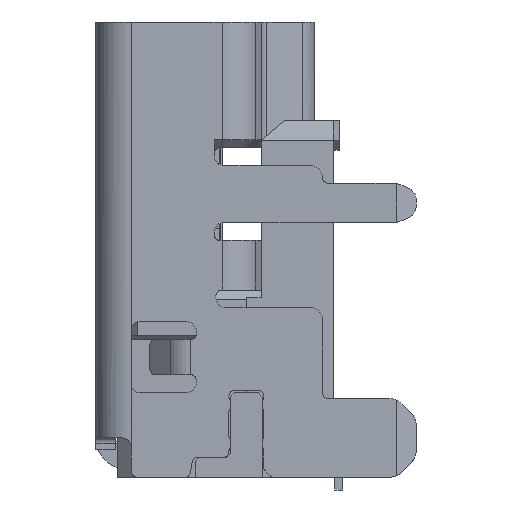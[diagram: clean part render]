
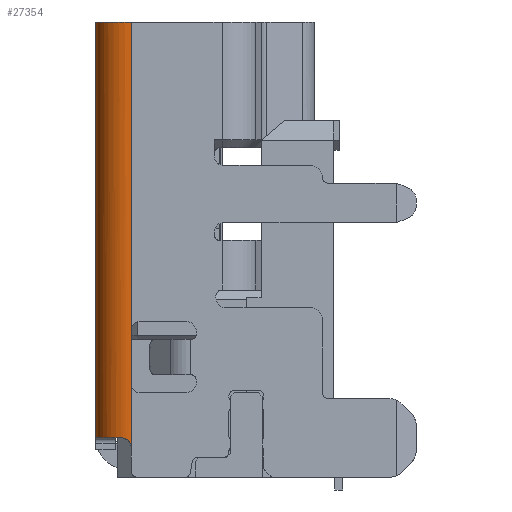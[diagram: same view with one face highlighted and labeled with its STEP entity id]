
A CAD part, left-side view. The second image highlights one B-rep face of the part: STEP entity #27354.
In plain terms, the highlighted cylindrical face has radius 0.9 mm (diameter 1.8 mm), a partial arc.
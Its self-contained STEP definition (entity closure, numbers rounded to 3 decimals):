
#1960 = DIRECTION ( 'NONE',  ( 0., 0., 1. ) ) ;
#2924 = VERTEX_POINT ( 'NONE', #66297 ) ;
#3146 = DIRECTION ( 'NONE',  ( 0., 0., -1. ) ) ;
#3292 = DIRECTION ( 'NONE',  ( 0., 0., -1. ) ) ;
#3440 = CARTESIAN_POINT ( 'NONE',  ( -7.5, -1.875, 2.42 ) ) ;
#4005 = AXIS2_PLACEMENT_3D ( 'NONE', #53851, #48777, #43670 ) ;
#4174 = CIRCLE ( 'NONE', #64042, 0.9 ) ;
#5714 = EDGE_CURVE ( 'NONE', #2924, #71550, #4174, .T. ) ;
#6759 = ORIENTED_EDGE ( 'NONE', *, *, #42271, .T. ) ;
#8764 = CARTESIAN_POINT ( 'NONE',  ( -7.5, -1.875, -1.005 ) ) ;
#10180 = EDGE_CURVE ( 'NONE', #45390, #64215, #56453, .T. ) ;
#12087 = CARTESIAN_POINT ( 'NONE',  ( -7.5, -1.875, 3.953 ) ) ;
#14672 = VECTOR ( 'NONE', #3146, 1000. ) ;
#15556 = VECTOR ( 'NONE', #62275, 1000. ) ;
#15806 = LINE ( 'NONE', #8764, #19588 ) ;
#19575 = CARTESIAN_POINT ( 'NONE',  ( -7.465, -2.125, 3.77 ) ) ;
#19588 = VECTOR ( 'NONE', #3292, 1000. ) ;
#20979 = DIRECTION ( 'NONE',  ( 0., 0., 1. ) ) ;
#22442 = CARTESIAN_POINT ( 'NONE',  ( -7.5, -1.875, 4.02 ) ) ;
#24005 = CIRCLE ( 'NONE', #4005, 0.9 ) ;
#25497 = CARTESIAN_POINT ( 'NONE',  ( -7.5, -1.875, -6.996 ) ) ;
#26940 = EDGE_CURVE ( 'NONE', #62517, #68354, #32882, .T. ) ;
#27354 = ADVANCED_FACE ( 'NONE', ( #62005 ), #57639, .T. ) ;
#28954 = CARTESIAN_POINT ( 'NONE',  ( -7.465, -2.125, 3.77 ) ) ;
#29230 = CARTESIAN_POINT ( 'NONE',  ( -6.6, -2.775, -6.78 ) ) ;
#29969 = ORIENTED_EDGE ( 'NONE', *, *, #5714, .T. ) ;
#30055 = DIRECTION ( 'NONE',  ( 0., 0., -1. ) ) ;
#31316 = ORIENTED_EDGE ( 'NONE', *, *, #49543, .T. ) ;
#32688 = CARTESIAN_POINT ( 'NONE',  ( -6.6, -1.875, -6.996 ) ) ;
#32882 = LINE ( 'NONE', #25497, #14672 ) ;
#33837 = DIRECTION ( 'NONE',  ( 1., 0., 0. ) ) ;
#35543 = CARTESIAN_POINT ( 'NONE',  ( -7.501, -1.903, 3.888 ) ) ;
#38303 = CARTESIAN_POINT ( 'NONE',  ( -6.6, -1.875, -6.78 ) ) ;
#39000 = EDGE_LOOP ( 'NONE', ( #59599, #59923, #70439, #31316, #29969, #6759, #40076 ) ) ;
#40076 = ORIENTED_EDGE ( 'NONE', *, *, #71233, .F. ) ;
#41010 = CARTESIAN_POINT ( 'NONE',  ( -7.483, -2.061, 3.77 ) ) ;
#42271 = EDGE_CURVE ( 'NONE', #71550, #43521, #44668, .T. ) ;
#43521 = VERTEX_POINT ( 'NONE', #47850 ) ;
#43670 = DIRECTION ( 'NONE',  ( 1., 0., 0. ) ) ;
#44668 = LINE ( 'NONE', #67747, #15556 ) ;
#45390 = VERTEX_POINT ( 'NONE', #19575 ) ;
#46478 = CARTESIAN_POINT ( 'NONE',  ( -7.5, -1.875, 4.02 ) ) ;
#47850 = CARTESIAN_POINT ( 'NONE',  ( -6.6, -2.775, 3.77 ) ) ;
#48777 = DIRECTION ( 'NONE',  ( 0., 0., 1. ) ) ;
#49543 = EDGE_CURVE ( 'NONE', #68354, #2924, #59683, .T. ) ;
#52723 = CARTESIAN_POINT ( 'NONE',  ( -7.493, -1.996, 3.796 ) ) ;
#53189 = AXIS2_PLACEMENT_3D ( 'NONE', #32688, #20979, #33837 ) ;
#53235 = VECTOR ( 'NONE', #30055, 1000. ) ;
#53851 = CARTESIAN_POINT ( 'NONE',  ( -6.6, -1.875, 3.77 ) ) ;
#56453 = B_SPLINE_CURVE_WITH_KNOTS ( 'NONE', 3,
 ( #28954, #41010, #52723, #35543, #12087, #46478 ),
 .UNSPECIFIED., .F., .F.,
 ( 4, 2, 4 ),
 ( 0., 0., 0. ),
 .UNSPECIFIED. ) ;
#57639 = CYLINDRICAL_SURFACE ( 'NONE', #53189, 0.9 ) ;
#58355 = CARTESIAN_POINT ( 'NONE',  ( -7.5, -1.875, 1.02 ) ) ;
#59599 = ORIENTED_EDGE ( 'NONE', *, *, #10180, .T. ) ;
#59683 = LINE ( 'NONE', #66338, #53235 ) ;
#59923 = ORIENTED_EDGE ( 'NONE', *, *, #62814, .T. ) ;
#62005 = FACE_OUTER_BOUND ( 'NONE', #39000, .T. ) ;
#62141 = DIRECTION ( 'NONE',  ( 1., 0., 0. ) ) ;
#62275 = DIRECTION ( 'NONE',  ( 0., 0., 1. ) ) ;
#62517 = VERTEX_POINT ( 'NONE', #3440 ) ;
#62814 = EDGE_CURVE ( 'NONE', #64215, #62517, #15806, .T. ) ;
#64042 = AXIS2_PLACEMENT_3D ( 'NONE', #38303, #1960, #62141 ) ;
#64215 = VERTEX_POINT ( 'NONE', #22442 ) ;
#66297 = CARTESIAN_POINT ( 'NONE',  ( -7.5, -1.875, -6.78 ) ) ;
#66338 = CARTESIAN_POINT ( 'NONE',  ( -7.5, -1.875, -6.996 ) ) ;
#67747 = CARTESIAN_POINT ( 'NONE',  ( -6.6, -2.775, -1.355 ) ) ;
#68354 = VERTEX_POINT ( 'NONE', #58355 ) ;
#70439 = ORIENTED_EDGE ( 'NONE', *, *, #26940, .T. ) ;
#71233 = EDGE_CURVE ( 'NONE', #45390, #43521, #24005, .T. ) ;
#71550 = VERTEX_POINT ( 'NONE', #29230 ) ;
